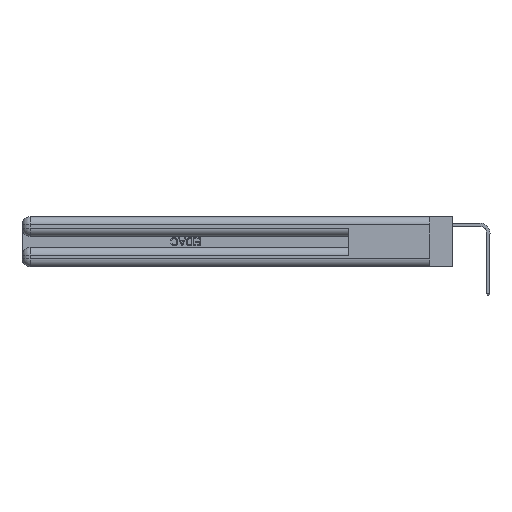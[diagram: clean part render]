
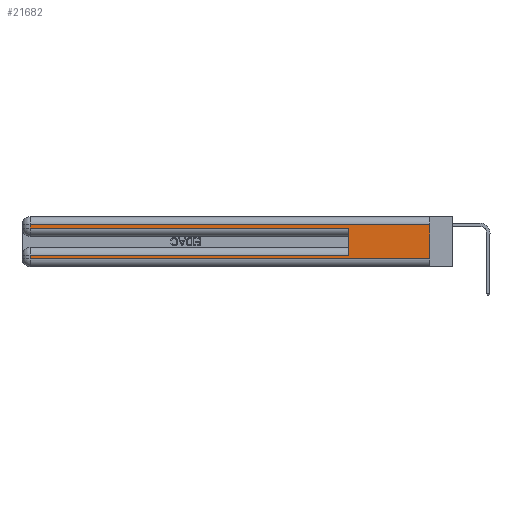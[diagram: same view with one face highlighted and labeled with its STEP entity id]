
A CAD part, left-side view. The second image highlights one B-rep face of the part: STEP entity #21682.
In plain terms, the highlighted planar face has unit normal (-1, 0, 0).
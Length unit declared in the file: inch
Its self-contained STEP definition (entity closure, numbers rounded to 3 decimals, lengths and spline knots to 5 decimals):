
#268 = DIRECTION ( 'NONE',  ( 0., 0., -1. ) ) ;
#771 = ORIENTED_EDGE ( 'NONE', *, *, #2204, .T. ) ;
#1056 = DIRECTION ( 'NONE',  ( 0., 1., 0. ) ) ;
#1880 = CARTESIAN_POINT ( 'NONE',  ( 0., 0., 0.285 ) ) ;
#2166 = EDGE_CURVE ( 'NONE', #12397, #4969, #22674, .T. ) ;
#2193 = ORIENTED_EDGE ( 'NONE', *, *, #5479, .T. ) ;
#2204 = EDGE_CURVE ( 'NONE', #10300, #3228, #27604, .T. ) ;
#2679 = CARTESIAN_POINT ( 'NONE',  ( 0., 2.94, 0.37 ) ) ;
#2919 = LINE ( 'NONE', #21254, #26483 ) ;
#3228 = VERTEX_POINT ( 'NONE', #8692 ) ;
#4244 = ORIENTED_EDGE ( 'NONE', *, *, #2166, .F. ) ;
#4501 = DIRECTION ( 'NONE',  ( 0., 1., 0. ) ) ;
#4969 = VERTEX_POINT ( 'NONE', #13790 ) ;
#5022 = DIRECTION ( 'NONE',  ( 0., 0., -1. ) ) ;
#5479 = EDGE_CURVE ( 'NONE', #9349, #13501, #19991, .T. ) ;
#6105 = EDGE_CURVE ( 'NONE', #3228, #16455, #27693, .T. ) ;
#6931 = VECTOR ( 'NONE', #1056, 39.37008 ) ;
#7655 = LINE ( 'NONE', #23862, #6931 ) ;
#7767 = DIRECTION ( 'NONE',  ( 0., -1., 0. ) ) ;
#8692 = CARTESIAN_POINT ( 'NONE',  ( 0., 2.94, 0.285 ) ) ;
#8929 = FACE_OUTER_BOUND ( 'NONE', #10341, .T. ) ;
#9162 = EDGE_CURVE ( 'NONE', #13501, #4969, #2919, .T. ) ;
#9349 = VERTEX_POINT ( 'NONE', #12878 ) ;
#9463 = VECTOR ( 'NONE', #5022, 39.37008 ) ;
#9560 = VECTOR ( 'NONE', #13238, 39.37008 ) ;
#9591 = EDGE_CURVE ( 'NONE', #22811, #9349, #26461, .T. ) ;
#10300 = VERTEX_POINT ( 'NONE', #12117 ) ;
#10341 = EDGE_LOOP ( 'NONE', ( #4244, #22764, #771, #20198, #26697, #28033, #2193, #23317 ) ) ;
#10612 = CARTESIAN_POINT ( 'NONE',  ( 0., 2.94, 0.06 ) ) ;
#10985 = LINE ( 'NONE', #17003, #22475 ) ;
#11380 = CARTESIAN_POINT ( 'NONE',  ( 0., 0., 0.085 ) ) ;
#11393 = EDGE_CURVE ( 'NONE', #22811, #16455, #10985, .T. ) ;
#12117 = CARTESIAN_POINT ( 'NONE',  ( 0., 2.94, 0.31 ) ) ;
#12397 = VERTEX_POINT ( 'NONE', #20809 ) ;
#12878 = CARTESIAN_POINT ( 'NONE',  ( 0., 2.94, 0.085 ) ) ;
#12931 = DIRECTION ( 'NONE',  ( 1., 0., 0. ) ) ;
#13238 = DIRECTION ( 'NONE',  ( 0., -1., 0. ) ) ;
#13501 = VERTEX_POINT ( 'NONE', #10612 ) ;
#13790 = CARTESIAN_POINT ( 'NONE',  ( 0., 0., 0.06 ) ) ;
#15050 = VECTOR ( 'NONE', #4501, 39.37008 ) ;
#16255 = CARTESIAN_POINT ( 'NONE',  ( 0., 0., 0.37 ) ) ;
#16293 = CARTESIAN_POINT ( 'NONE',  ( 0., 0.6, 0.285 ) ) ;
#16455 = VERTEX_POINT ( 'NONE', #16293 ) ;
#17003 = CARTESIAN_POINT ( 'NONE',  ( 0., 0.6, 0.145 ) ) ;
#19345 = DIRECTION ( 'NONE',  ( 0., 0., 1. ) ) ;
#19991 = LINE ( 'NONE', #24967, #24578 ) ;
#20198 = ORIENTED_EDGE ( 'NONE', *, *, #6105, .T. ) ;
#20809 = CARTESIAN_POINT ( 'NONE',  ( 0., 0., 0.31 ) ) ;
#21254 = CARTESIAN_POINT ( 'NONE',  ( 0., 0., 0.06 ) ) ;
#21682 = ADVANCED_FACE ( 'NONE', ( #8929 ), #23269, .F. ) ;
#22475 = VECTOR ( 'NONE', #19345, 39.37008 ) ;
#22674 = LINE ( 'NONE', #16255, #27916 ) ;
#22764 = ORIENTED_EDGE ( 'NONE', *, *, #26453, .T. ) ;
#22811 = VERTEX_POINT ( 'NONE', #26143 ) ;
#23269 = PLANE ( 'NONE',  #28555 ) ;
#23317 = ORIENTED_EDGE ( 'NONE', *, *, #9162, .T. ) ;
#23862 = CARTESIAN_POINT ( 'NONE',  ( 0., 0., 0.31 ) ) ;
#24578 = VECTOR ( 'NONE', #27204, 39.37008 ) ;
#24967 = CARTESIAN_POINT ( 'NONE',  ( 0., 2.94, 0.37 ) ) ;
#26143 = CARTESIAN_POINT ( 'NONE',  ( 0., 0.6, 0.085 ) ) ;
#26453 = EDGE_CURVE ( 'NONE', #12397, #10300, #7655, .T. ) ;
#26461 = LINE ( 'NONE', #11380, #15050 ) ;
#26483 = VECTOR ( 'NONE', #7767, 39.37008 ) ;
#26582 = CARTESIAN_POINT ( 'NONE',  ( 0., 0., 0.37 ) ) ;
#26697 = ORIENTED_EDGE ( 'NONE', *, *, #11393, .F. ) ;
#27204 = DIRECTION ( 'NONE',  ( 0., 0., -1. ) ) ;
#27604 = LINE ( 'NONE', #2679, #9463 ) ;
#27693 = LINE ( 'NONE', #1880, #9560 ) ;
#27916 = VECTOR ( 'NONE', #268, 39.37008 ) ;
#28033 = ORIENTED_EDGE ( 'NONE', *, *, #9591, .T. ) ;
#28555 = AXIS2_PLACEMENT_3D ( 'NONE', #26582, #12931, #28852 ) ;
#28852 = DIRECTION ( 'NONE',  ( 0., 0., -1. ) ) ;
